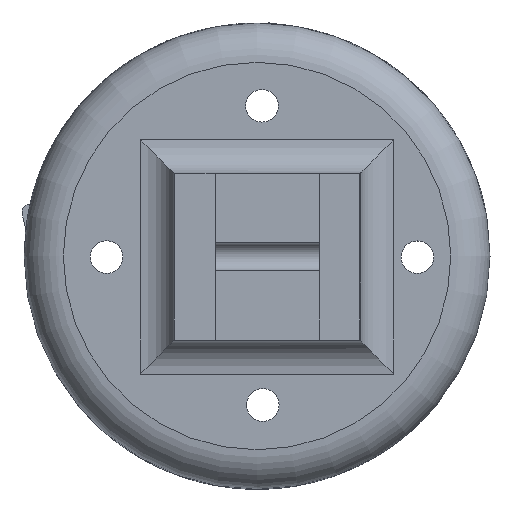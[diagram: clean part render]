
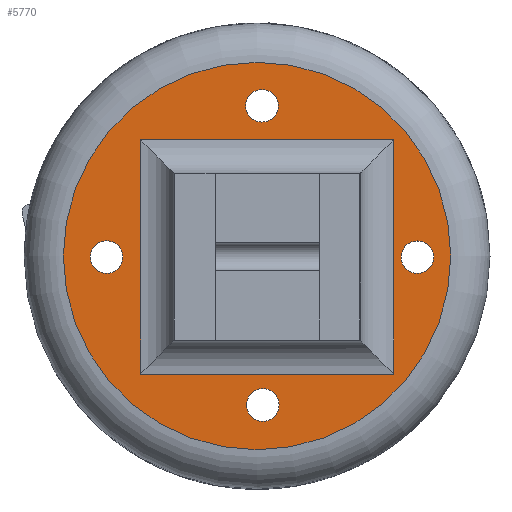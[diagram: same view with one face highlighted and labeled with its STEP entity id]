
A CAD part, top view. The second image highlights one B-rep face of the part: STEP entity #5770.
In plain terms, the highlighted face is planar.
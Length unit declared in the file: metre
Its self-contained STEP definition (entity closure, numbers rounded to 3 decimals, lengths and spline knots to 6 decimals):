
#5770=ADVANCED_FACE('0:6016',(#11714,#11715,#11716,#11717,#11718,#11719),#11720,.T.);
#11714=FACE_BOUND('',#43521,.T.);
#11715=FACE_BOUND('',#43522,.T.);
#11716=FACE_BOUND('',#43523,.T.);
#11717=FACE_BOUND('',#43524,.T.);
#11718=FACE_OUTER_BOUND('',#43525,.T.);
#11719=FACE_BOUND('',#43526,.T.);
#11720=PLANE('',#43527);
#43521=EDGE_LOOP('',(#60737,#60738));
#43522=EDGE_LOOP('',(#60739,#60740));
#43523=EDGE_LOOP('',(#60741,#60742));
#43524=EDGE_LOOP('',(#60743,#60744));
#43525=EDGE_LOOP('',(#60745,#60746));
#43526=EDGE_LOOP('',(#60747,#60748,#60749,#60750));
#43527=AXIS2_PLACEMENT_3D('',#60751,#60752,#60753);
#60737=ORIENTED_EDGE('',*,*,#71049,.T.);
#60738=ORIENTED_EDGE('',*,*,#71050,.T.);
#60739=ORIENTED_EDGE('',*,*,#71051,.T.);
#60740=ORIENTED_EDGE('',*,*,#71052,.T.);
#60741=ORIENTED_EDGE('',*,*,#71053,.T.);
#60742=ORIENTED_EDGE('',*,*,#71054,.T.);
#60743=ORIENTED_EDGE('',*,*,#71055,.T.);
#60744=ORIENTED_EDGE('',*,*,#71056,.T.);
#60745=ORIENTED_EDGE('',*,*,#71057,.F.);
#60746=ORIENTED_EDGE('',*,*,#71058,.F.);
#60747=ORIENTED_EDGE('',*,*,#71059,.F.);
#60748=ORIENTED_EDGE('',*,*,#71060,.F.);
#60749=ORIENTED_EDGE('',*,*,#71061,.F.);
#60750=ORIENTED_EDGE('',*,*,#71062,.F.);
#60751=CARTESIAN_POINT('',(-0.046289,0.038136,-0.00226));
#60752=DIRECTION('',(0.0,0.,-1.0));
#60753=DIRECTION('',(-1.0,0.0,0.0));
#71049=EDGE_CURVE('0:6114',#92893,#92894,#92895,.T.);
#71050=EDGE_CURVE('0:6114',#92894,#92893,#92896,.T.);
#71051=EDGE_CURVE('0:6108',#92897,#92898,#92899,.T.);
#71052=EDGE_CURVE('0:6108',#92898,#92897,#92900,.T.);
#71053=EDGE_CURVE('0:6102',#92901,#92902,#92903,.T.);
#71054=EDGE_CURVE('0:6102',#92902,#92901,#92904,.T.);
#71055=EDGE_CURVE('0:6096',#92905,#92906,#92907,.T.);
#71056=EDGE_CURVE('0:6096',#92906,#92905,#92908,.T.);
#71057=EDGE_CURVE('0:20337',#92909,#92910,#92911,.T.);
#71058=EDGE_CURVE('0:20337',#92910,#92909,#92912,.T.);
#71059=EDGE_CURVE('6:4333',#92913,#92914,#92915,.T.);
#71060=EDGE_CURVE('6:4348',#92916,#92913,#92917,.T.);
#71061=EDGE_CURVE('6:4342',#92918,#92916,#92919,.T.);
#71062=EDGE_CURVE('6:4339',#92914,#92918,#92920,.T.);
#92893=VERTEX_POINT('',#131779);
#92894=VERTEX_POINT('',#131780);
#92895=CIRCLE('',#131781,0.002481);
#92896=CIRCLE('',#131782,0.002481);
#92897=VERTEX_POINT('',#131783);
#92898=VERTEX_POINT('',#131784);
#92899=CIRCLE('',#131785,0.002481);
#92900=CIRCLE('',#131786,0.002481);
#92901=VERTEX_POINT('',#131787);
#92902=VERTEX_POINT('',#131788);
#92903=CIRCLE('',#131789,0.002481);
#92904=CIRCLE('',#131790,0.002481);
#92905=VERTEX_POINT('',#131791);
#92906=VERTEX_POINT('',#131792);
#92907=CIRCLE('',#131793,0.002481);
#92908=CIRCLE('',#131794,0.002481);
#92909=VERTEX_POINT('',#131795);
#92910=VERTEX_POINT('',#131796);
#92911=CIRCLE('',#131797,0.029505);
#92912=CIRCLE('',#131798,0.029505);
#92913=VERTEX_POINT('',#131799);
#92914=VERTEX_POINT('',#131800);
#92915=LINE('',#131801,#131802);
#92916=VERTEX_POINT('',#131803);
#92917=LINE('',#131804,#131805);
#92918=VERTEX_POINT('',#131806);
#92919=LINE('',#131807,#131808);
#92920=LINE('',#131809,#131810);
#131779=CARTESIAN_POINT('',(-0.071684,0.03829,-0.00226));
#131780=CARTESIAN_POINT('',(-0.066723,0.03829,-0.00226));
#131781=AXIS2_PLACEMENT_3D('',#140152,#140153,#140154);
#131782=AXIS2_PLACEMENT_3D('',#140155,#140156,#140157);
#131783=CARTESIAN_POINT('',(-0.047905,0.060826,-0.00226));
#131784=CARTESIAN_POINT('',(-0.042943,0.060826,-0.00226));
#131785=AXIS2_PLACEMENT_3D('',#140158,#140159,#140160);
#131786=AXIS2_PLACEMENT_3D('',#140161,#140162,#140163);
#131787=CARTESIAN_POINT('',(-0.024356,0.038324,-0.00226));
#131788=CARTESIAN_POINT('',(-0.019394,0.038324,-0.00226));
#131789=AXIS2_PLACEMENT_3D('',#140164,#140165,#140166);
#131790=AXIS2_PLACEMENT_3D('',#140167,#140168,#140169);
#131791=CARTESIAN_POINT('',(-0.048022,0.015254,-0.00226));
#131792=CARTESIAN_POINT('',(-0.04306,0.015254,-0.00226));
#131793=AXIS2_PLACEMENT_3D('',#140170,#140171,#140172);
#131794=AXIS2_PLACEMENT_3D('',#140173,#140174,#140175);
#131795=CARTESIAN_POINT('',(-0.075794,0.038136,-0.00226));
#131796=CARTESIAN_POINT('',(-0.016785,0.038136,-0.00226));
#131797=AXIS2_PLACEMENT_3D('',#140176,#140177,#140178);
#131798=AXIS2_PLACEMENT_3D('',#140179,#140180,#140181);
#131799=CARTESIAN_POINT('',(-0.025479,0.020435,-0.00226));
#131800=CARTESIAN_POINT('',(-0.064035,0.020435,-0.00226));
#131801=CARTESIAN_POINT('',(-0.04478,0.020435,-0.00226));
#131802=VECTOR('',#140182,1.0);
#131803=CARTESIAN_POINT('',(-0.025479,0.05611,-0.00226));
#131804=CARTESIAN_POINT('',(-0.025479,0.038273,-0.00226));
#131805=VECTOR('',#140183,1.0);
#131806=CARTESIAN_POINT('',(-0.064035,0.05611,-0.00226));
#131807=CARTESIAN_POINT('',(-0.04478,0.05611,-0.00226));
#131808=VECTOR('',#140184,1.0);
#131809=CARTESIAN_POINT('',(-0.064035,0.038273,-0.00226));
#131810=VECTOR('',#140185,1.0);
#140152=CARTESIAN_POINT('',(-0.069203,0.03829,-0.00226));
#140153=DIRECTION('',(0.0,0.,1.0));
#140154=DIRECTION('',(1.0,0.0,0.0));
#140155=CARTESIAN_POINT('',(-0.069203,0.03829,-0.00226));
#140156=DIRECTION('',(0.0,0.,1.0));
#140157=DIRECTION('',(1.0,0.0,0.0));
#140158=CARTESIAN_POINT('',(-0.045424,0.060826,-0.00226));
#140159=DIRECTION('',(0.0,0.,1.0));
#140160=DIRECTION('',(1.0,0.0,0.0));
#140161=CARTESIAN_POINT('',(-0.045424,0.060826,-0.00226));
#140162=DIRECTION('',(0.0,0.,1.0));
#140163=DIRECTION('',(1.0,0.0,0.0));
#140164=CARTESIAN_POINT('',(-0.021875,0.038324,-0.00226));
#140165=DIRECTION('',(0.0,0.,1.0));
#140166=DIRECTION('',(1.0,0.0,0.0));
#140167=CARTESIAN_POINT('',(-0.021875,0.038324,-0.00226));
#140168=DIRECTION('',(0.0,0.,1.0));
#140169=DIRECTION('',(1.0,0.0,0.0));
#140170=CARTESIAN_POINT('',(-0.045541,0.015254,-0.00226));
#140171=DIRECTION('',(0.0,0.,1.0));
#140172=DIRECTION('',(1.0,0.0,0.0));
#140173=CARTESIAN_POINT('',(-0.045541,0.015254,-0.00226));
#140174=DIRECTION('',(0.0,0.,1.0));
#140175=DIRECTION('',(1.0,0.0,0.0));
#140176=CARTESIAN_POINT('',(-0.046289,0.038136,-0.00226));
#140177=DIRECTION('',(0.,0.,1.0));
#140178=DIRECTION('',(1.0,0.,0.));
#140179=CARTESIAN_POINT('',(-0.046289,0.038136,-0.00226));
#140180=DIRECTION('',(0.,0.,1.0));
#140181=DIRECTION('',(1.0,0.,0.));
#140182=DIRECTION('',(-1.0,0.,0.));
#140183=DIRECTION('',(0.,-1.0,0.));
#140184=DIRECTION('',(1.0,0.,0.));
#140185=DIRECTION('',(0.,1.0,0.));
